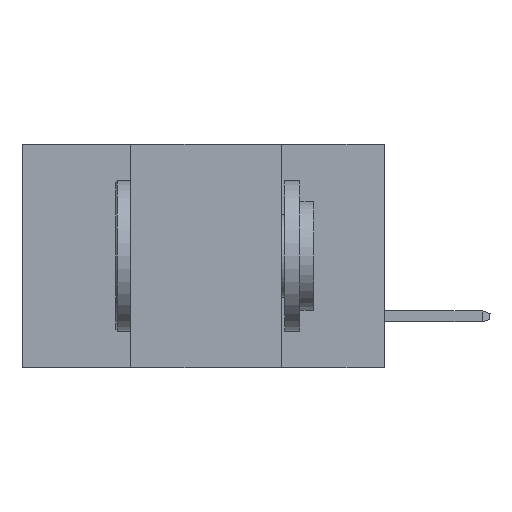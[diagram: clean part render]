
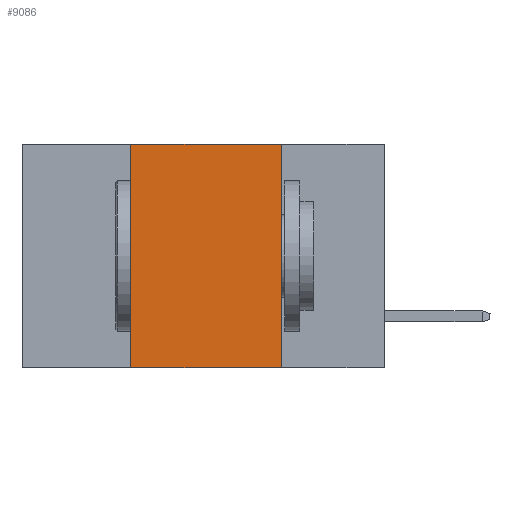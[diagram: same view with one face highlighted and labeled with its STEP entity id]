
A CAD part, left-side view. The second image highlights one B-rep face of the part: STEP entity #9086.
In plain terms, the highlighted planar face has unit normal (-1, 0, 0).
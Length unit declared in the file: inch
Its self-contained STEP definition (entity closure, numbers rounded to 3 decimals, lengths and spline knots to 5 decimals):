
#55 = CARTESIAN_POINT ( 'NONE',  ( 0., 0.17, 0. ) ) ;
#201 = VECTOR ( 'NONE', #12914, 39.37008 ) ;
#499 = PLANE ( 'NONE',  #10598 ) ;
#1522 = LINE ( 'NONE', #6441, #6417 ) ;
#1711 = DIRECTION ( 'NONE',  ( 1., 0., 0. ) ) ;
#2961 = EDGE_CURVE ( 'NONE', #11723, #6037, #1522, .T. ) ;
#4205 = EDGE_CURVE ( 'NONE', #11723, #7099, #4271, .T. ) ;
#4271 = LINE ( 'NONE', #5314, #201 ) ;
#5309 = DIRECTION ( 'NONE',  ( 0., 0., -1. ) ) ;
#5314 = CARTESIAN_POINT ( 'NONE',  ( 0., 0.6, -0.37 ) ) ;
#5966 = CARTESIAN_POINT ( 'NONE',  ( 0., 0.17, -0.37 ) ) ;
#6037 = VERTEX_POINT ( 'NONE', #7168 ) ;
#6359 = LINE ( 'NONE', #9674, #12938 ) ;
#6417 = VECTOR ( 'NONE', #11375, 39.37008 ) ;
#6441 = CARTESIAN_POINT ( 'NONE',  ( 0., 0.42, -0.37 ) ) ;
#6700 = CARTESIAN_POINT ( 'NONE',  ( 0., 0.6, 0. ) ) ;
#7099 = VERTEX_POINT ( 'NONE', #5966 ) ;
#7168 = CARTESIAN_POINT ( 'NONE',  ( 0., 0.42, 0. ) ) ;
#7326 = EDGE_CURVE ( 'NONE', #6037, #10216, #6359, .T. ) ;
#7407 = DIRECTION ( 'NONE',  ( 0., -1., 0. ) ) ;
#8287 = ORIENTED_EDGE ( 'NONE', *, *, #7326, .F. ) ;
#9086 = ADVANCED_FACE ( 'NONE', ( #10506 ), #499, .F. ) ;
#9153 = CARTESIAN_POINT ( 'NONE',  ( 0., 0.42, -0.37 ) ) ;
#9511 = EDGE_CURVE ( 'NONE', #10216, #7099, #11697, .T. ) ;
#9674 = CARTESIAN_POINT ( 'NONE',  ( 0., 0.6, 0. ) ) ;
#10044 = VECTOR ( 'NONE', #5309, 39.37008 ) ;
#10216 = VERTEX_POINT ( 'NONE', #55 ) ;
#10350 = DIRECTION ( 'NONE',  ( 0., 0., -1. ) ) ;
#10506 = FACE_OUTER_BOUND ( 'NONE', #14364, .T. ) ;
#10598 = AXIS2_PLACEMENT_3D ( 'NONE', #6700, #1711, #10350 ) ;
#11375 = DIRECTION ( 'NONE',  ( 0., 0., 1. ) ) ;
#11697 = LINE ( 'NONE', #12989, #10044 ) ;
#11723 = VERTEX_POINT ( 'NONE', #9153 ) ;
#11863 = ORIENTED_EDGE ( 'NONE', *, *, #4205, .T. ) ;
#12914 = DIRECTION ( 'NONE',  ( 0., -1., 0. ) ) ;
#12938 = VECTOR ( 'NONE', #7407, 39.37008 ) ;
#12989 = CARTESIAN_POINT ( 'NONE',  ( 0., 0.17, -0.37 ) ) ;
#13967 = ORIENTED_EDGE ( 'NONE', *, *, #2961, .F. ) ;
#14364 = EDGE_LOOP ( 'NONE', ( #14528, #8287, #13967, #11863 ) ) ;
#14528 = ORIENTED_EDGE ( 'NONE', *, *, #9511, .F. ) ;
